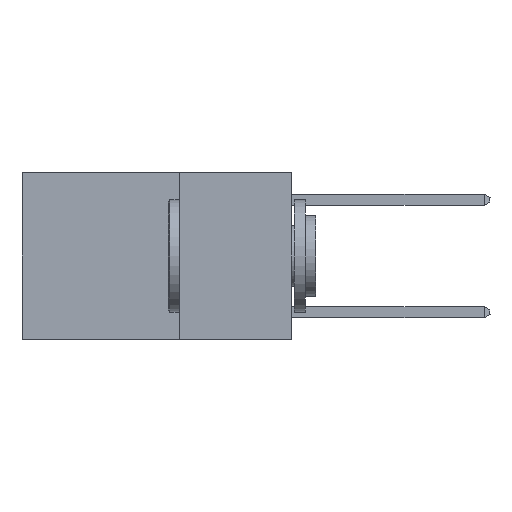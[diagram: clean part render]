
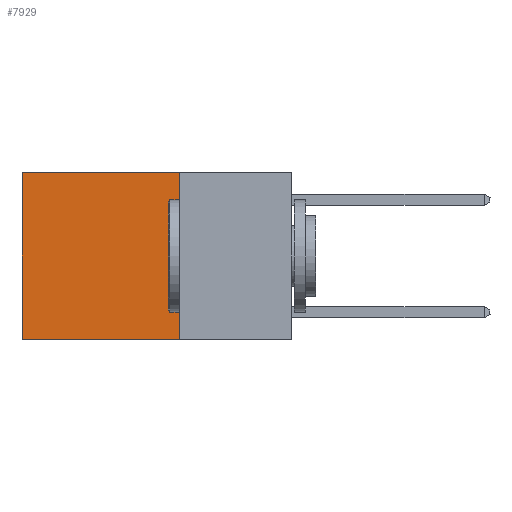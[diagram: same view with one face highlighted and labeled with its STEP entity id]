
A CAD part, left-side view. The second image highlights one B-rep face of the part: STEP entity #7929.
In plain terms, the highlighted planar face has unit normal (-1, 0, 0).
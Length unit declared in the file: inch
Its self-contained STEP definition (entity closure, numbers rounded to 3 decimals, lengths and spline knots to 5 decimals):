
#1369 = LINE ( 'NONE', #23965, #1436 ) ;
#1436 = VECTOR ( 'NONE', #22365, 39.37008 ) ;
#2215 = AXIS2_PLACEMENT_3D ( 'NONE', #14127, #21644, #11740 ) ;
#3365 = LINE ( 'NONE', #19863, #12436 ) ;
#4039 = EDGE_CURVE ( 'NONE', #14284, #12270, #12349, .T. ) ;
#4925 = EDGE_CURVE ( 'NONE', #6766, #18660, #1369, .T. ) ;
#4999 = CARTESIAN_POINT ( 'NONE',  ( 0.2625, 0.25, -0.37 ) ) ;
#5039 = CARTESIAN_POINT ( 'NONE',  ( 0.2625, 0.6, -0.37 ) ) ;
#5632 = ORIENTED_EDGE ( 'NONE', *, *, #9712, .F. ) ;
#6626 = PLANE ( 'NONE',  #2215 ) ;
#6719 = CARTESIAN_POINT ( 'NONE',  ( 0.2625, 0.25, 0. ) ) ;
#6766 = VERTEX_POINT ( 'NONE', #4999 ) ;
#7929 = ADVANCED_FACE ( 'NONE', ( #23507 ), #6626, .F. ) ;
#8279 = CARTESIAN_POINT ( 'NONE',  ( 0.2625, 0.25, 0. ) ) ;
#8833 = EDGE_CURVE ( 'NONE', #12270, #18660, #3365, .T. ) ;
#8903 = DIRECTION ( 'NONE',  ( 0., 0., -1. ) ) ;
#9692 = VECTOR ( 'NONE', #12225, 39.37008 ) ;
#9712 = EDGE_CURVE ( 'NONE', #14284, #6766, #12508, .T. ) ;
#9935 = ORIENTED_EDGE ( 'NONE', *, *, #8833, .T. ) ;
#11740 = DIRECTION ( 'NONE',  ( 0., 0., -1. ) ) ;
#12225 = DIRECTION ( 'NONE',  ( 0., 1., 0. ) ) ;
#12270 = VERTEX_POINT ( 'NONE', #21546 ) ;
#12349 = LINE ( 'NONE', #8279, #9692 ) ;
#12436 = VECTOR ( 'NONE', #8903, 39.37008 ) ;
#12508 = LINE ( 'NONE', #6719, #22191 ) ;
#14127 = CARTESIAN_POINT ( 'NONE',  ( 0.2625, 0.25, 0. ) ) ;
#14284 = VERTEX_POINT ( 'NONE', #17529 ) ;
#17529 = CARTESIAN_POINT ( 'NONE',  ( 0.2625, 0.25, 0. ) ) ;
#17941 = EDGE_LOOP ( 'NONE', ( #9935, #21223, #5632, #22106 ) ) ;
#18660 = VERTEX_POINT ( 'NONE', #5039 ) ;
#19863 = CARTESIAN_POINT ( 'NONE',  ( 0.2625, 0.6, 0. ) ) ;
#20022 = DIRECTION ( 'NONE',  ( 0., 0., -1. ) ) ;
#21223 = ORIENTED_EDGE ( 'NONE', *, *, #4925, .F. ) ;
#21546 = CARTESIAN_POINT ( 'NONE',  ( 0.2625, 0.6, 0. ) ) ;
#21644 = DIRECTION ( 'NONE',  ( 1., 0., 0. ) ) ;
#22106 = ORIENTED_EDGE ( 'NONE', *, *, #4039, .T. ) ;
#22191 = VECTOR ( 'NONE', #20022, 39.37008 ) ;
#22365 = DIRECTION ( 'NONE',  ( 0., 1., 0. ) ) ;
#23507 = FACE_OUTER_BOUND ( 'NONE', #17941, .T. ) ;
#23965 = CARTESIAN_POINT ( 'NONE',  ( 0.2625, 0.25, -0.37 ) ) ;
